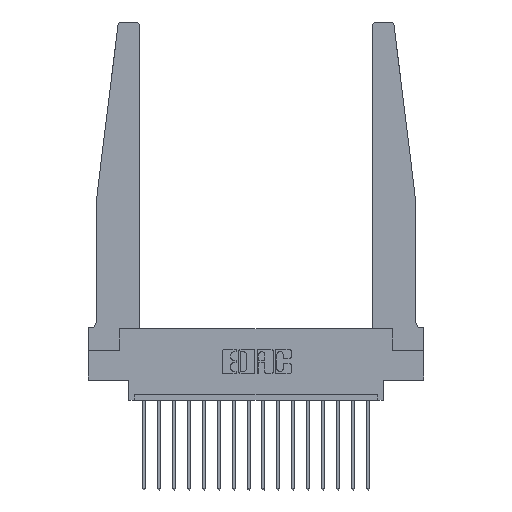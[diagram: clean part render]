
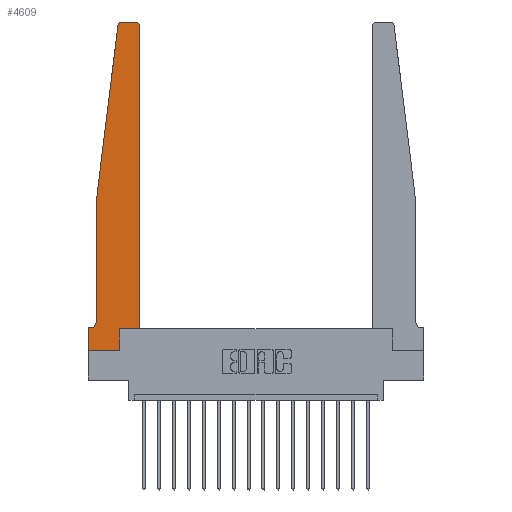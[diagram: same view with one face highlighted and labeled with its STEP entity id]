
A CAD part, top view. The second image highlights one B-rep face of the part: STEP entity #4609.
In plain terms, the highlighted planar face has unit normal (0, 0, 1).
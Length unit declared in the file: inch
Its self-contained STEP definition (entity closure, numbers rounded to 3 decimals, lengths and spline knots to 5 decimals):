
#88 = EDGE_CURVE ( 'NONE', #8410, #16923, #1833, .T. ) ;
#664 = DIRECTION ( 'NONE',  ( 1., 0., 0. ) ) ;
#924 = CARTESIAN_POINT ( 'NONE',  ( 0.24675, 2.72367, 0.37 ) ) ;
#1021 = CARTESIAN_POINT ( 'NONE',  ( 0.015, 0.1875, 0.37 ) ) ;
#1036 = LINE ( 'NONE', #6469, #9630 ) ;
#1127 = VECTOR ( 'NONE', #8546, 39.37008 ) ;
#1327 = DIRECTION ( 'NONE',  ( 1., 0., 0. ) ) ;
#1365 = VERTEX_POINT ( 'NONE', #11681 ) ;
#1519 = DIRECTION ( 'NONE',  ( 0., -1., 0. ) ) ;
#1807 = EDGE_CURVE ( 'NONE', #14783, #8410, #5700, .T. ) ;
#1833 = LINE ( 'NONE', #8993, #1127 ) ;
#2173 = DIRECTION ( 'NONE',  ( 0., 0., 1. ) ) ;
#2436 = ORIENTED_EDGE ( 'NONE', *, *, #5591, .T. ) ;
#2477 = DIRECTION ( 'NONE',  ( 0., 1., 0. ) ) ;
#2642 = CIRCLE ( 'NONE', #8348, 0.03 ) ;
#2802 = VERTEX_POINT ( 'NONE', #8009 ) ;
#3018 = VECTOR ( 'NONE', #10616, 39.37008 ) ;
#3231 = DIRECTION ( 'NONE',  ( 0., -1., 0. ) ) ;
#3447 = LINE ( 'NONE', #8814, #3018 ) ;
#3596 = ORIENTED_EDGE ( 'NONE', *, *, #15472, .T. ) ;
#3779 = ORIENTED_EDGE ( 'NONE', *, *, #13549, .T. ) ;
#4123 = AXIS2_PLACEMENT_3D ( 'NONE', #10654, #10822, #6305 ) ;
#4609 = ADVANCED_FACE ( 'NONE', ( #9155 ), #13796, .T. ) ;
#4768 = DIRECTION ( 'NONE',  ( 0., 1., 0. ) ) ;
#4938 = CARTESIAN_POINT ( 'NONE',  ( 0., 0.1875, 0.37 ) ) ;
#5099 = ORIENTED_EDGE ( 'NONE', *, *, #16436, .T. ) ;
#5105 = VERTEX_POINT ( 'NONE', #6384 ) ;
#5119 = DIRECTION ( 'NONE',  ( 1., 0., 0. ) ) ;
#5145 = LINE ( 'NONE', #10709, #17837 ) ;
#5534 = VERTEX_POINT ( 'NONE', #924 ) ;
#5591 = EDGE_CURVE ( 'NONE', #10403, #6537, #6574, .T. ) ;
#5700 = LINE ( 'NONE', #11663, #10951 ) ;
#6305 = DIRECTION ( 'NONE',  ( -1., 0., 0. ) ) ;
#6319 = DIRECTION ( 'NONE',  ( 0., 0., 1. ) ) ;
#6384 = CARTESIAN_POINT ( 'NONE',  ( 0.425, 0.18, 0.37 ) ) ;
#6469 = CARTESIAN_POINT ( 'NONE',  ( 0.2605, 0.18, 0.37 ) ) ;
#6537 = VERTEX_POINT ( 'NONE', #16539 ) ;
#6574 = LINE ( 'NONE', #10744, #17363 ) ;
#6945 = VERTEX_POINT ( 'NONE', #1021 ) ;
#7213 = AXIS2_PLACEMENT_3D ( 'NONE', #4938, #2173, #5119 ) ;
#7691 = EDGE_CURVE ( 'NONE', #5105, #17096, #5145, .T. ) ;
#8009 = CARTESIAN_POINT ( 'NONE',  ( 0.2605, 0.18, 0.37 ) ) ;
#8279 = VECTOR ( 'NONE', #14353, 39.37008 ) ;
#8319 = ORIENTED_EDGE ( 'NONE', *, *, #17417, .T. ) ;
#8348 = AXIS2_PLACEMENT_3D ( 'NONE', #12872, #11478, #1327 ) ;
#8410 = VERTEX_POINT ( 'NONE', #15882 ) ;
#8525 = ORIENTED_EDGE ( 'NONE', *, *, #9622, .T. ) ;
#8546 = DIRECTION ( 'NONE',  ( 1., 0., 0. ) ) ;
#8814 = CARTESIAN_POINT ( 'NONE',  ( 0.25, 2.75, 0.37 ) ) ;
#8993 = CARTESIAN_POINT ( 'NONE',  ( 0., 0., 0.37 ) ) ;
#9155 = FACE_OUTER_BOUND ( 'NONE', #13243, .T. ) ;
#9409 = EDGE_CURVE ( 'NONE', #16923, #2802, #1036, .T. ) ;
#9542 = CIRCLE ( 'NONE', #4123, 0.05 ) ;
#9622 = EDGE_CURVE ( 'NONE', #15421, #1365, #3447, .T. ) ;
#9630 = VECTOR ( 'NONE', #2477, 39.37008 ) ;
#9726 = CARTESIAN_POINT ( 'NONE',  ( 0.065, 0.1875, 0.37 ) ) ;
#9812 = DIRECTION ( 'NONE',  ( -1., 0., 0. ) ) ;
#10227 = ORIENTED_EDGE ( 'NONE', *, *, #1807, .T. ) ;
#10403 = VERTEX_POINT ( 'NONE', #11294 ) ;
#10616 = DIRECTION ( 'NONE',  ( -1., 0., 0. ) ) ;
#10654 = CARTESIAN_POINT ( 'NONE',  ( 0.015, 0.2375, 0.37 ) ) ;
#10709 = CARTESIAN_POINT ( 'NONE',  ( 0.425, 0.18, 0.37 ) ) ;
#10710 = CARTESIAN_POINT ( 'NONE',  ( 0.425, 0.18, 0.37 ) ) ;
#10744 = CARTESIAN_POINT ( 'NONE',  ( 0.065, 1.25, 0.37 ) ) ;
#10748 = CARTESIAN_POINT ( 'NONE',  ( 0.395, 2.72, 0.37 ) ) ;
#10822 = DIRECTION ( 'NONE',  ( 0., 0., -1. ) ) ;
#10951 = VECTOR ( 'NONE', #1519, 39.37008 ) ;
#11294 = CARTESIAN_POINT ( 'NONE',  ( 0.065, 1.25, 0.37 ) ) ;
#11415 = LINE ( 'NONE', #13977, #8279 ) ;
#11478 = DIRECTION ( 'NONE',  ( 0., 0., 1. ) ) ;
#11663 = CARTESIAN_POINT ( 'NONE',  ( 0., 0., 0.37 ) ) ;
#11681 = CARTESIAN_POINT ( 'NONE',  ( 0.27653, 2.75, 0.37 ) ) ;
#11755 = CARTESIAN_POINT ( 'NONE',  ( 0.395, 2.75, 0.37 ) ) ;
#12235 = LINE ( 'NONE', #9726, #13275 ) ;
#12872 = CARTESIAN_POINT ( 'NONE',  ( 0.27653, 2.72, 0.37 ) ) ;
#12935 = AXIS2_PLACEMENT_3D ( 'NONE', #10748, #6319, #14743 ) ;
#13209 = EDGE_CURVE ( 'NONE', #5534, #10403, #11415, .T. ) ;
#13243 = EDGE_LOOP ( 'NONE', ( #8525, #3596, #16758, #2436, #3779, #8319, #10227, #17149, #13659, #14124, #16712, #5099 ) ) ;
#13275 = VECTOR ( 'NONE', #9812, 39.37008 ) ;
#13549 = EDGE_CURVE ( 'NONE', #6537, #6945, #9542, .T. ) ;
#13659 = ORIENTED_EDGE ( 'NONE', *, *, #9409, .T. ) ;
#13771 = CARTESIAN_POINT ( 'NONE',  ( 0., 0.1875, 0.37 ) ) ;
#13796 = PLANE ( 'NONE',  #7213 ) ;
#13977 = CARTESIAN_POINT ( 'NONE',  ( 0.065, 1.25, 0.37 ) ) ;
#14124 = ORIENTED_EDGE ( 'NONE', *, *, #17395, .T. ) ;
#14353 = DIRECTION ( 'NONE',  ( -0.122, -0.992, 0. ) ) ;
#14508 = CARTESIAN_POINT ( 'NONE',  ( 0.425, 2.72, 0.37 ) ) ;
#14743 = DIRECTION ( 'NONE',  ( 1., 0., 0. ) ) ;
#14783 = VERTEX_POINT ( 'NONE', #13771 ) ;
#15421 = VERTEX_POINT ( 'NONE', #11755 ) ;
#15472 = EDGE_CURVE ( 'NONE', #1365, #5534, #2642, .T. ) ;
#15675 = CIRCLE ( 'NONE', #12935, 0.03 ) ;
#15718 = LINE ( 'NONE', #10710, #18749 ) ;
#15882 = CARTESIAN_POINT ( 'NONE',  ( 0., 0., 0.37 ) ) ;
#16436 = EDGE_CURVE ( 'NONE', #17096, #15421, #15675, .T. ) ;
#16539 = CARTESIAN_POINT ( 'NONE',  ( 0.065, 0.2375, 0.37 ) ) ;
#16712 = ORIENTED_EDGE ( 'NONE', *, *, #7691, .T. ) ;
#16758 = ORIENTED_EDGE ( 'NONE', *, *, #13209, .T. ) ;
#16923 = VERTEX_POINT ( 'NONE', #18341 ) ;
#17096 = VERTEX_POINT ( 'NONE', #14508 ) ;
#17149 = ORIENTED_EDGE ( 'NONE', *, *, #88, .T. ) ;
#17363 = VECTOR ( 'NONE', #3231, 39.37008 ) ;
#17395 = EDGE_CURVE ( 'NONE', #2802, #5105, #15718, .T. ) ;
#17417 = EDGE_CURVE ( 'NONE', #6945, #14783, #12235, .T. ) ;
#17837 = VECTOR ( 'NONE', #4768, 39.37008 ) ;
#18341 = CARTESIAN_POINT ( 'NONE',  ( 0.2605, 0., 0.37 ) ) ;
#18749 = VECTOR ( 'NONE', #664, 39.37008 ) ;
